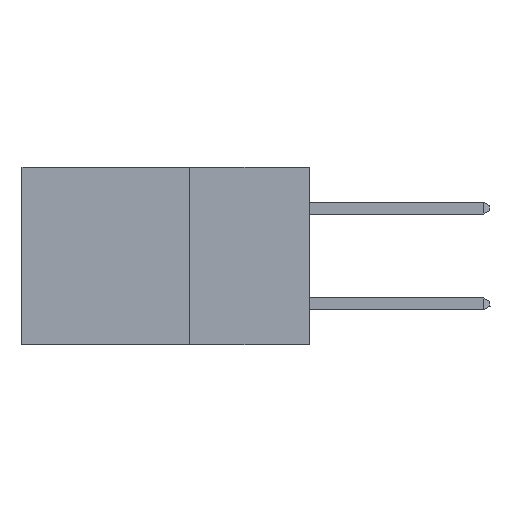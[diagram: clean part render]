
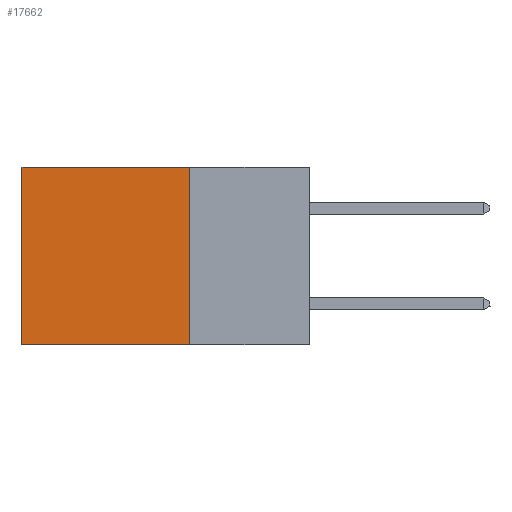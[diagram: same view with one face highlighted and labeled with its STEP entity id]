
A CAD part, left-side view. The second image highlights one B-rep face of the part: STEP entity #17662.
In plain terms, the highlighted planar face has unit normal (-1, 0, 0).
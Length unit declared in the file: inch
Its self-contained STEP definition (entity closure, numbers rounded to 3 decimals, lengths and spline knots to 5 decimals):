
#847 = DIRECTION ( 'NONE',  ( 0., 0., -1. ) ) ;
#857 = LINE ( 'NONE', #23567, #13084 ) ;
#1397 = CARTESIAN_POINT ( 'NONE',  ( 0.2875, 0.25, 0. ) ) ;
#1745 = LINE ( 'NONE', #9164, #8580 ) ;
#3313 = DIRECTION ( 'NONE',  ( 0., 1., 0. ) ) ;
#5369 = CARTESIAN_POINT ( 'NONE',  ( 0.2875, 0.25, 0. ) ) ;
#6619 = EDGE_CURVE ( 'NONE', #27387, #26250, #30919, .T. ) ;
#6916 = ORIENTED_EDGE ( 'NONE', *, *, #13227, .T. ) ;
#7143 = EDGE_LOOP ( 'NONE', ( #6916, #13002, #14428, #27879 ) ) ;
#8078 = EDGE_CURVE ( 'NONE', #14561, #29807, #1745, .T. ) ;
#8580 = VECTOR ( 'NONE', #14056, 39.37008 ) ;
#9164 = CARTESIAN_POINT ( 'NONE',  ( 0.2875, 0.25, -0.37 ) ) ;
#10714 = CARTESIAN_POINT ( 'NONE',  ( 0.2875, 0.25, -0.37 ) ) ;
#11492 = EDGE_CURVE ( 'NONE', #27387, #14561, #22790, .T. ) ;
#12773 = CARTESIAN_POINT ( 'NONE',  ( 0.2875, 0.25, 0. ) ) ;
#13002 = ORIENTED_EDGE ( 'NONE', *, *, #8078, .F. ) ;
#13084 = VECTOR ( 'NONE', #26349, 39.37008 ) ;
#13227 = EDGE_CURVE ( 'NONE', #26250, #29807, #857, .T. ) ;
#13732 = PLANE ( 'NONE',  #22610 ) ;
#14056 = DIRECTION ( 'NONE',  ( 0., 1., 0. ) ) ;
#14428 = ORIENTED_EDGE ( 'NONE', *, *, #11492, .F. ) ;
#14561 = VERTEX_POINT ( 'NONE', #10714 ) ;
#17662 = ADVANCED_FACE ( 'NONE', ( #27372 ), #13732, .F. ) ;
#18521 = DIRECTION ( 'NONE',  ( 1., 0., 0. ) ) ;
#22610 = AXIS2_PLACEMENT_3D ( 'NONE', #1397, #18521, #25891 ) ;
#22689 = CARTESIAN_POINT ( 'NONE',  ( 0.2875, 0.6, 0. ) ) ;
#22790 = LINE ( 'NONE', #12773, #24684 ) ;
#23567 = CARTESIAN_POINT ( 'NONE',  ( 0.2875, 0.6, 0. ) ) ;
#23630 = VECTOR ( 'NONE', #3313, 39.37008 ) ;
#24211 = CARTESIAN_POINT ( 'NONE',  ( 0.2875, 0.25, 0. ) ) ;
#24684 = VECTOR ( 'NONE', #847, 39.37008 ) ;
#25891 = DIRECTION ( 'NONE',  ( 0., 0., -1. ) ) ;
#26250 = VERTEX_POINT ( 'NONE', #22689 ) ;
#26349 = DIRECTION ( 'NONE',  ( 0., 0., -1. ) ) ;
#27372 = FACE_OUTER_BOUND ( 'NONE', #7143, .T. ) ;
#27387 = VERTEX_POINT ( 'NONE', #5369 ) ;
#27744 = CARTESIAN_POINT ( 'NONE',  ( 0.2875, 0.6, -0.37 ) ) ;
#27879 = ORIENTED_EDGE ( 'NONE', *, *, #6619, .T. ) ;
#29807 = VERTEX_POINT ( 'NONE', #27744 ) ;
#30919 = LINE ( 'NONE', #24211, #23630 ) ;
